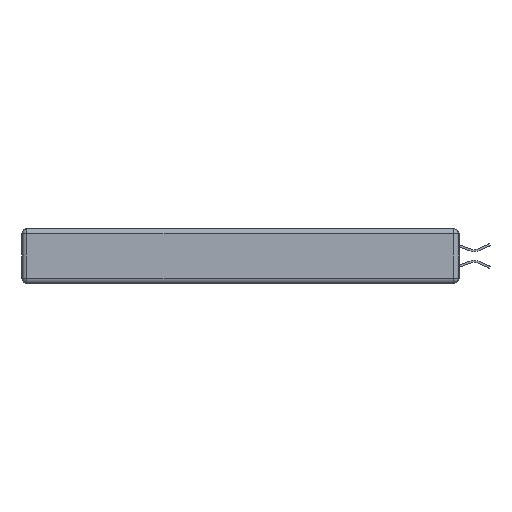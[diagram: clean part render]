
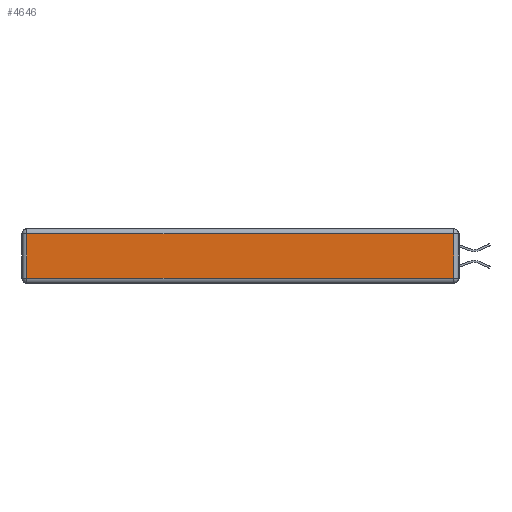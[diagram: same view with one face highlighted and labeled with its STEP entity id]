
A CAD part, left-side view. The second image highlights one B-rep face of the part: STEP entity #4646.
In plain terms, the highlighted planar face has unit normal (-1, 0, 0).
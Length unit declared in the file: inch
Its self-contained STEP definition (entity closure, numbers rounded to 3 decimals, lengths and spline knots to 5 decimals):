
#457 = EDGE_CURVE ( 'NONE', #19571, #9403, #14786, .T. ) ;
#1799 = DIRECTION ( 'NONE',  ( 0., 1., 0. ) ) ;
#2744 = VERTEX_POINT ( 'NONE', #10415 ) ;
#2881 = EDGE_CURVE ( 'NONE', #9403, #18006, #6137, .T. ) ;
#3397 = CARTESIAN_POINT ( 'NONE',  ( 0., 0.03, -0.313 ) ) ;
#3760 = EDGE_CURVE ( 'NONE', #18006, #2744, #5534, .T. ) ;
#3852 = ORIENTED_EDGE ( 'NONE', *, *, #3760, .T. ) ;
#4030 = CARTESIAN_POINT ( 'NONE',  ( 0., 0., -0.343 ) ) ;
#4413 = EDGE_CURVE ( 'NONE', #2744, #19571, #14161, .T. ) ;
#4646 = ADVANCED_FACE ( 'NONE', ( #17518 ), #13995, .T. ) ;
#4758 = AXIS2_PLACEMENT_3D ( 'NONE', #4030, #10810, #15657 ) ;
#5534 = LINE ( 'NONE', #8564, #18550 ) ;
#6086 = ORIENTED_EDGE ( 'NONE', *, *, #2881, .T. ) ;
#6137 = LINE ( 'NONE', #12775, #10294 ) ;
#7402 = CARTESIAN_POINT ( 'NONE',  ( 0., 2.72, -0.313 ) ) ;
#8564 = CARTESIAN_POINT ( 'NONE',  ( 0., 0.03, -0.343 ) ) ;
#9403 = VERTEX_POINT ( 'NONE', #7402 ) ;
#10294 = VECTOR ( 'NONE', #21254, 39.37008 ) ;
#10379 = VECTOR ( 'NONE', #14844, 39.37008 ) ;
#10415 = CARTESIAN_POINT ( 'NONE',  ( 0., 0.03, -0.03 ) ) ;
#10810 = DIRECTION ( 'NONE',  ( -1., 0., 0. ) ) ;
#11982 = CARTESIAN_POINT ( 'NONE',  ( 0., 2.75, -0.03 ) ) ;
#12273 = ORIENTED_EDGE ( 'NONE', *, *, #4413, .T. ) ;
#12385 = CARTESIAN_POINT ( 'NONE',  ( 0., 2.72, -0.03 ) ) ;
#12775 = CARTESIAN_POINT ( 'NONE',  ( 0., 0., -0.313 ) ) ;
#13995 = PLANE ( 'NONE',  #4758 ) ;
#14161 = LINE ( 'NONE', #11982, #19607 ) ;
#14450 = ORIENTED_EDGE ( 'NONE', *, *, #457, .T. ) ;
#14786 = LINE ( 'NONE', #16271, #10379 ) ;
#14844 = DIRECTION ( 'NONE',  ( 0., 0., -1. ) ) ;
#14944 = EDGE_LOOP ( 'NONE', ( #6086, #3852, #12273, #14450 ) ) ;
#15284 = DIRECTION ( 'NONE',  ( 0., 0., 1. ) ) ;
#15657 = DIRECTION ( 'NONE',  ( 0., 0., 1. ) ) ;
#16271 = CARTESIAN_POINT ( 'NONE',  ( 0., 2.72, -0.343 ) ) ;
#17518 = FACE_OUTER_BOUND ( 'NONE', #14944, .T. ) ;
#18006 = VERTEX_POINT ( 'NONE', #3397 ) ;
#18550 = VECTOR ( 'NONE', #15284, 39.37008 ) ;
#19571 = VERTEX_POINT ( 'NONE', #12385 ) ;
#19607 = VECTOR ( 'NONE', #1799, 39.37008 ) ;
#21254 = DIRECTION ( 'NONE',  ( 0., -1., 0. ) ) ;
